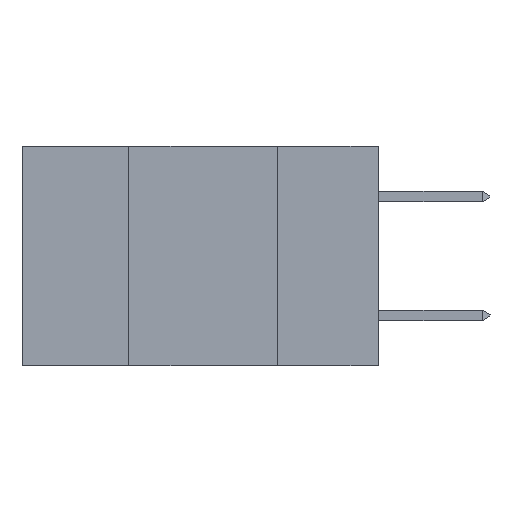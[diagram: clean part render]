
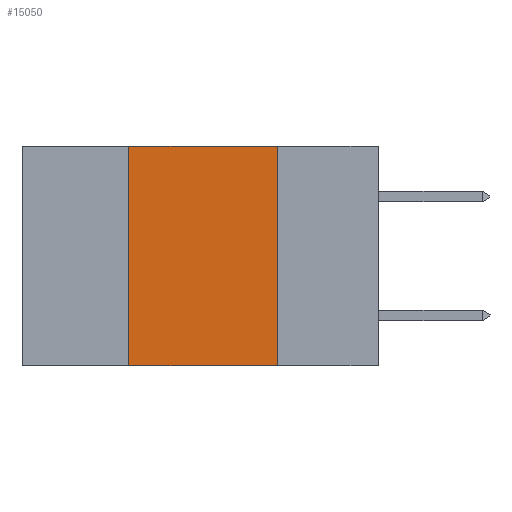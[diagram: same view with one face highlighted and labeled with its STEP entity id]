
A CAD part, left-side view. The second image highlights one B-rep face of the part: STEP entity #15050.
In plain terms, the highlighted planar face has unit normal (-1, 0, 0).
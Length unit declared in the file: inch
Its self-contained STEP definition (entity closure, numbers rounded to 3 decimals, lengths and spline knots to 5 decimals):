
#179 = DIRECTION ( 'NONE',  ( 0., 0., -1. ) ) ;
#894 = LINE ( 'NONE', #24146, #11741 ) ;
#1983 = ORIENTED_EDGE ( 'NONE', *, *, #14542, .T. ) ;
#2467 = LINE ( 'NONE', #2990, #16935 ) ;
#2990 = CARTESIAN_POINT ( 'NONE',  ( 0., 0.6, -0.37 ) ) ;
#3220 = AXIS2_PLACEMENT_3D ( 'NONE', #28306, #15127, #179 ) ;
#3467 = VECTOR ( 'NONE', #19816, 39.37008 ) ;
#4234 = VERTEX_POINT ( 'NONE', #12386 ) ;
#8415 = ORIENTED_EDGE ( 'NONE', *, *, #32794, .F. ) ;
#8696 = DIRECTION ( 'NONE',  ( 0., 0., -1. ) ) ;
#8728 = CARTESIAN_POINT ( 'NONE',  ( 0., 0.42, 0. ) ) ;
#9952 = VERTEX_POINT ( 'NONE', #32064 ) ;
#10822 = VECTOR ( 'NONE', #16489, 39.37008 ) ;
#10971 = DIRECTION ( 'NONE',  ( 0., -1., 0. ) ) ;
#11741 = VECTOR ( 'NONE', #8696, 39.37008 ) ;
#12386 = CARTESIAN_POINT ( 'NONE',  ( 0., 0.17, -0.37 ) ) ;
#12694 = EDGE_CURVE ( 'NONE', #31042, #9952, #23740, .T. ) ;
#14542 = EDGE_CURVE ( 'NONE', #25085, #4234, #2467, .T. ) ;
#15050 = ADVANCED_FACE ( 'NONE', ( #22562 ), #31018, .F. ) ;
#15127 = DIRECTION ( 'NONE',  ( 1., 0., 0. ) ) ;
#16489 = DIRECTION ( 'NONE',  ( 0., -1., 0. ) ) ;
#16935 = VECTOR ( 'NONE', #10971, 39.37008 ) ;
#19571 = LINE ( 'NONE', #19701, #3467 ) ;
#19701 = CARTESIAN_POINT ( 'NONE',  ( 0., 0.42, 0. ) ) ;
#19816 = DIRECTION ( 'NONE',  ( 0., 0., 1. ) ) ;
#21811 = EDGE_CURVE ( 'NONE', #25085, #31042, #19571, .T. ) ;
#22183 = CARTESIAN_POINT ( 'NONE',  ( 0., 0.42, -0.37 ) ) ;
#22562 = FACE_OUTER_BOUND ( 'NONE', #26074, .T. ) ;
#23518 = ORIENTED_EDGE ( 'NONE', *, *, #12694, .F. ) ;
#23740 = LINE ( 'NONE', #29362, #10822 ) ;
#24146 = CARTESIAN_POINT ( 'NONE',  ( 0., 0.17, 0. ) ) ;
#25085 = VERTEX_POINT ( 'NONE', #22183 ) ;
#26074 = EDGE_LOOP ( 'NONE', ( #8415, #23518, #26123, #1983 ) ) ;
#26123 = ORIENTED_EDGE ( 'NONE', *, *, #21811, .F. ) ;
#28306 = CARTESIAN_POINT ( 'NONE',  ( 0., 0.6, 0. ) ) ;
#29362 = CARTESIAN_POINT ( 'NONE',  ( 0., 0.6, 0. ) ) ;
#31018 = PLANE ( 'NONE',  #3220 ) ;
#31042 = VERTEX_POINT ( 'NONE', #8728 ) ;
#32064 = CARTESIAN_POINT ( 'NONE',  ( 0., 0.17, 0. ) ) ;
#32794 = EDGE_CURVE ( 'NONE', #9952, #4234, #894, .T. ) ;
